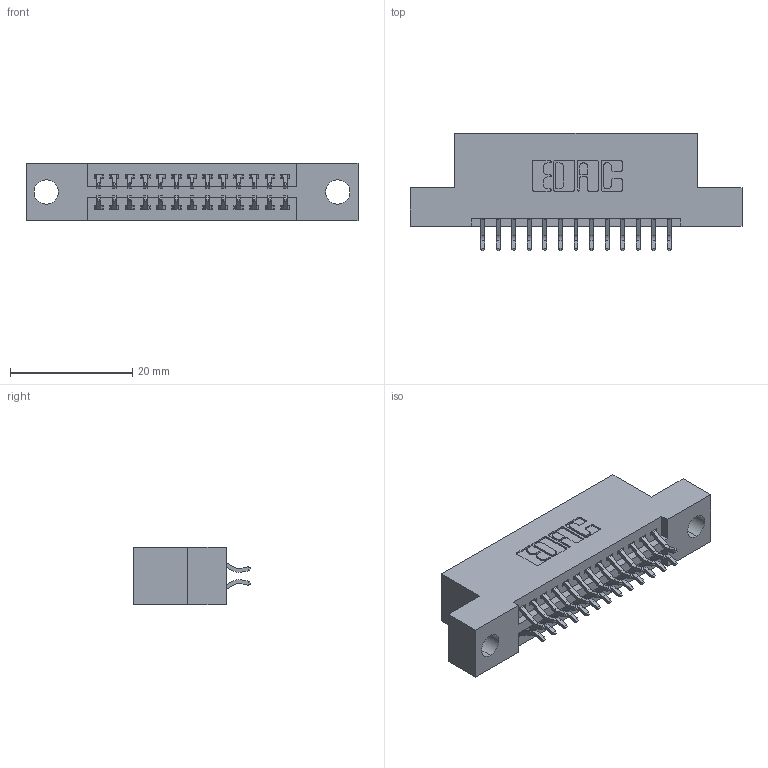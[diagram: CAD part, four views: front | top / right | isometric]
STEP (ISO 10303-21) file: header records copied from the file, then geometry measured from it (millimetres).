
FILE_DESCRIPTION (( 'STEP AP203' ), '1' );
FILE_NAME ('395-026-556-204.STEP', '2018-11-10T01:08:51', ( '' ), ( '' ), 'SwSTEP 2.0', 'SolidWorks 2016', '' );
FILE_SCHEMA (( 'CONFIG_CONTROL_DESIGN' ));
Length unit declared in the file: inch
Products named in the file (3): 345-292-001_556 Tail; 395-026-556-204; 345 Part_Flush Mounting Lugs - 0.156 Dia-TH
Assembly tree (27 placements, depth 2):
  395-026-556-204
    345 Part_Flush Mounting Lugs - 0.156 Dia-TH
    345-292-001_556 Tail  x26
Bounding box: 54.23 x 19.24 x 9.4 mm (x, y, z)
Volume: 4909.8 mm3; surface area: 6488.2 mm2
Topology: 27 solids, 27 shells, 1582 faces, 4683 edges, 3086 vertices
Faces by surface type: plane 1042, cylinder 540
Entity records: 14327 total; most frequent: CARTESIAN_POINT 2444, ORIENTED_EDGE 2366, DIRECTION 2179, EDGE_CURVE 1183, LINE 991, VECTOR 991, VERTEX_POINT 786, AXIS2_PLACEMENT_3D 594
